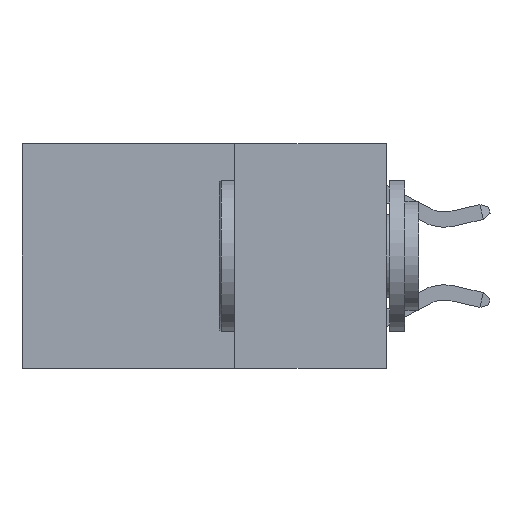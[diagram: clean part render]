
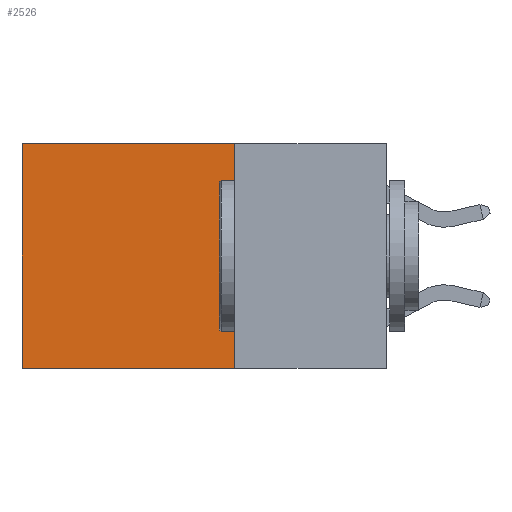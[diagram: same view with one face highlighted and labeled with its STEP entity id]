
A CAD part, left-side view. The second image highlights one B-rep face of the part: STEP entity #2526.
In plain terms, the highlighted planar face has unit normal (-1, 0, 0).
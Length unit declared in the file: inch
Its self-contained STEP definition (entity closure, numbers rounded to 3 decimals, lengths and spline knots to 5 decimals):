
#201 = DIRECTION ( 'NONE',  ( 0., 0., -1. ) ) ;
#202 = VERTEX_POINT ( 'NONE', #15575 ) ;
#490 = ORIENTED_EDGE ( 'NONE', *, *, #4799, .T. ) ;
#2503 = FACE_OUTER_BOUND ( 'NONE', #3904, .T. ) ;
#2526 = ADVANCED_FACE ( 'NONE', ( #2503 ), #16899, .F. ) ;
#3904 = EDGE_LOOP ( 'NONE', ( #490, #9808, #14967, #19618 ) ) ;
#4799 = EDGE_CURVE ( 'NONE', #7090, #16244, #21994, .T. ) ;
#5701 = VERTEX_POINT ( 'NONE', #21875 ) ;
#6463 = CARTESIAN_POINT ( 'NONE',  ( 0.2625, 0.25, 0. ) ) ;
#6650 = LINE ( 'NONE', #18457, #19988 ) ;
#7090 = VERTEX_POINT ( 'NONE', #10115 ) ;
#8220 = DIRECTION ( 'NONE',  ( 1., 0., 0. ) ) ;
#8756 = CARTESIAN_POINT ( 'NONE',  ( 0.2625, 0.6, -0.37 ) ) ;
#9242 = LINE ( 'NONE', #12046, #17948 ) ;
#9341 = VECTOR ( 'NONE', #20769, 39.37008 ) ;
#9808 = ORIENTED_EDGE ( 'NONE', *, *, #16183, .F. ) ;
#10115 = CARTESIAN_POINT ( 'NONE',  ( 0.2625, 0.6, 0. ) ) ;
#12046 = CARTESIAN_POINT ( 'NONE',  ( 0.2625, 0.25, 0. ) ) ;
#13275 = VECTOR ( 'NONE', #201, 39.37008 ) ;
#13786 = DIRECTION ( 'NONE',  ( 0., 1., 0. ) ) ;
#13937 = LINE ( 'NONE', #17278, #9341 ) ;
#14967 = ORIENTED_EDGE ( 'NONE', *, *, #21101, .F. ) ;
#15575 = CARTESIAN_POINT ( 'NONE',  ( 0.2625, 0.25, -0.37 ) ) ;
#16183 = EDGE_CURVE ( 'NONE', #202, #16244, #13937, .T. ) ;
#16244 = VERTEX_POINT ( 'NONE', #8756 ) ;
#16899 = PLANE ( 'NONE',  #22068 ) ;
#17278 = CARTESIAN_POINT ( 'NONE',  ( 0.2625, 0.25, -0.37 ) ) ;
#17948 = VECTOR ( 'NONE', #13786, 39.37008 ) ;
#18457 = CARTESIAN_POINT ( 'NONE',  ( 0.2625, 0.25, 0. ) ) ;
#18503 = EDGE_CURVE ( 'NONE', #5701, #7090, #9242, .T. ) ;
#19382 = CARTESIAN_POINT ( 'NONE',  ( 0.2625, 0.6, 0. ) ) ;
#19618 = ORIENTED_EDGE ( 'NONE', *, *, #18503, .T. ) ;
#19988 = VECTOR ( 'NONE', #20197, 39.37008 ) ;
#20197 = DIRECTION ( 'NONE',  ( 0., 0., -1. ) ) ;
#20392 = DIRECTION ( 'NONE',  ( 0., 0., -1. ) ) ;
#20769 = DIRECTION ( 'NONE',  ( 0., 1., 0. ) ) ;
#21101 = EDGE_CURVE ( 'NONE', #5701, #202, #6650, .T. ) ;
#21875 = CARTESIAN_POINT ( 'NONE',  ( 0.2625, 0.25, 0. ) ) ;
#21994 = LINE ( 'NONE', #19382, #13275 ) ;
#22068 = AXIS2_PLACEMENT_3D ( 'NONE', #6463, #8220, #20392 ) ;
